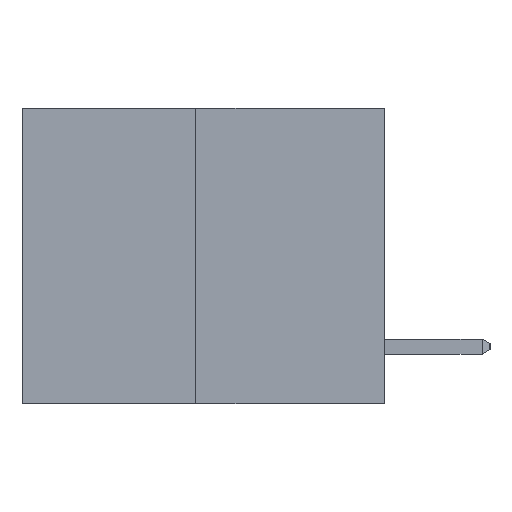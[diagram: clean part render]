
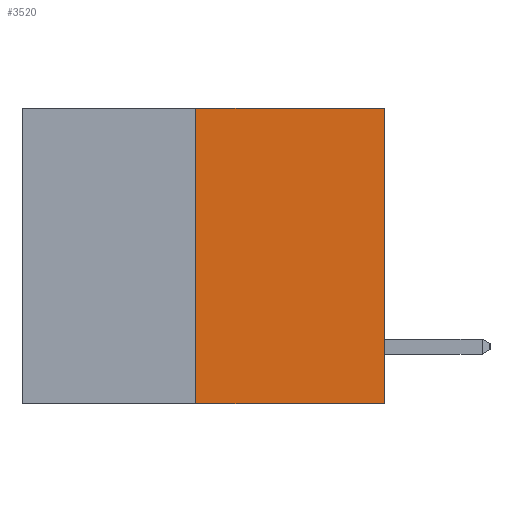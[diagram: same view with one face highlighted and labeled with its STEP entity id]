
A CAD part, left-side view. The second image highlights one B-rep face of the part: STEP entity #3520.
In plain terms, the highlighted planar face has unit normal (-1, 0, 0).
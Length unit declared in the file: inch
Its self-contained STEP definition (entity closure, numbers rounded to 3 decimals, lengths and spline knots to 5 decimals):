
#298 = CARTESIAN_POINT ( 'NONE',  ( 0., 0.312, -0.49 ) ) ;
#591 = EDGE_CURVE ( 'NONE', #3936, #15383, #17272, .T. ) ;
#618 = EDGE_CURVE ( 'NONE', #3936, #9733, #3103, .T. ) ;
#712 = LINE ( 'NONE', #17552, #7100 ) ;
#887 = CARTESIAN_POINT ( 'NONE',  ( 0., 0.6, -0.49 ) ) ;
#2182 = CARTESIAN_POINT ( 'NONE',  ( 0., 0.6, 0. ) ) ;
#2190 = EDGE_CURVE ( 'NONE', #9733, #12701, #712, .T. ) ;
#3103 = LINE ( 'NONE', #887, #15961 ) ;
#3261 = EDGE_LOOP ( 'NONE', ( #14983, #11188, #11461, #8531 ) ) ;
#3520 = ADVANCED_FACE ( 'NONE', ( #11366 ), #8799, .F. ) ;
#3936 = VERTEX_POINT ( 'NONE', #298 ) ;
#4915 = DIRECTION ( 'NONE',  ( 0., -1., 0. ) ) ;
#4973 = DIRECTION ( 'NONE',  ( 0., 0., 1. ) ) ;
#5236 = DIRECTION ( 'NONE',  ( 0., 0., 1. ) ) ;
#7100 = VECTOR ( 'NONE', #5236, 39.37008 ) ;
#7742 = CARTESIAN_POINT ( 'NONE',  ( 0., 0., 0. ) ) ;
#7956 = CARTESIAN_POINT ( 'NONE',  ( 0., 0., -0.49 ) ) ;
#8531 = ORIENTED_EDGE ( 'NONE', *, *, #13307, .F. ) ;
#8799 = PLANE ( 'NONE',  #17171 ) ;
#8848 = DIRECTION ( 'NONE',  ( 1., 0., 0. ) ) ;
#9120 = VECTOR ( 'NONE', #4973, 39.37008 ) ;
#9134 = DIRECTION ( 'NONE',  ( 0., -1., 0. ) ) ;
#9733 = VERTEX_POINT ( 'NONE', #7956 ) ;
#11188 = ORIENTED_EDGE ( 'NONE', *, *, #618, .T. ) ;
#11366 = FACE_OUTER_BOUND ( 'NONE', #3261, .T. ) ;
#11461 = ORIENTED_EDGE ( 'NONE', *, *, #2190, .T. ) ;
#12701 = VERTEX_POINT ( 'NONE', #7742 ) ;
#13275 = VECTOR ( 'NONE', #9134, 39.37008 ) ;
#13307 = EDGE_CURVE ( 'NONE', #15383, #12701, #16922, .T. ) ;
#14983 = ORIENTED_EDGE ( 'NONE', *, *, #591, .F. ) ;
#15383 = VERTEX_POINT ( 'NONE', #16591 ) ;
#15442 = DIRECTION ( 'NONE',  ( 0., 0., -1. ) ) ;
#15961 = VECTOR ( 'NONE', #4915, 39.37008 ) ;
#16591 = CARTESIAN_POINT ( 'NONE',  ( 0., 0.312, 0. ) ) ;
#16922 = LINE ( 'NONE', #2182, #13275 ) ;
#17068 = CARTESIAN_POINT ( 'NONE',  ( 0., 0.6, 0. ) ) ;
#17171 = AXIS2_PLACEMENT_3D ( 'NONE', #17068, #8848, #15442 ) ;
#17272 = LINE ( 'NONE', #17422, #9120 ) ;
#17422 = CARTESIAN_POINT ( 'NONE',  ( 0., 0.312, -0.49 ) ) ;
#17552 = CARTESIAN_POINT ( 'NONE',  ( 0., 0., 0. ) ) ;
